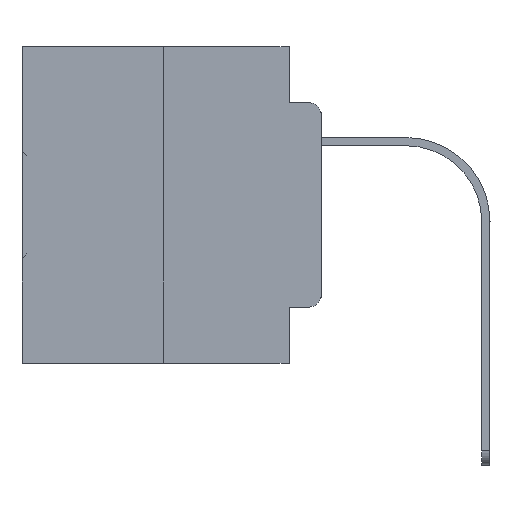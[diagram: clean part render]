
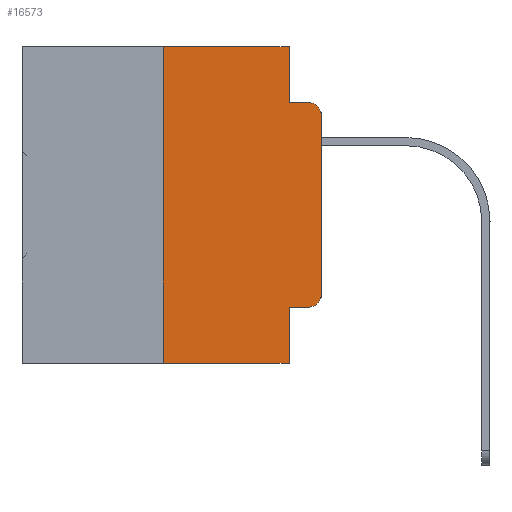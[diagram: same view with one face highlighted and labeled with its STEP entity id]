
A CAD part, left-side view. The second image highlights one B-rep face of the part: STEP entity #16573.
In plain terms, the highlighted planar face has unit normal (-1, 0, 0).
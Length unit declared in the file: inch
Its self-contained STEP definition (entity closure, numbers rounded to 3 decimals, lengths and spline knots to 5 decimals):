
#8 = ORIENTED_EDGE ( 'NONE', *, *, #15113, .F. ) ;
#86 = CIRCLE ( 'NONE', #32238, 0.02 ) ;
#237 = LINE ( 'NONE', #5363, #12974 ) ;
#696 = CARTESIAN_POINT ( 'NONE',  ( 0., 0.02, -0.1085 ) ) ;
#784 = VECTOR ( 'NONE', #29828, 39.37008 ) ;
#1221 = DIRECTION ( 'NONE',  ( -1., 0., 0. ) ) ;
#1241 = VERTEX_POINT ( 'NONE', #31182 ) ;
#1507 = VERTEX_POINT ( 'NONE', #30000 ) ;
#2081 = FACE_OUTER_BOUND ( 'NONE', #9160, .T. ) ;
#2321 = VECTOR ( 'NONE', #7804, 39.37008 ) ;
#2793 = EDGE_CURVE ( 'NONE', #11692, #13692, #12373, .T. ) ;
#2879 = ORIENTED_EDGE ( 'NONE', *, *, #31612, .T. ) ;
#3747 = DIRECTION ( 'NONE',  ( 0., 0., -1. ) ) ;
#4838 = AXIS2_PLACEMENT_3D ( 'NONE', #11300, #1221, #3747 ) ;
#5363 = CARTESIAN_POINT ( 'NONE',  ( 0., 0.051, -0.0885 ) ) ;
#6650 = CARTESIAN_POINT ( 'NONE',  ( 0., 0.25, 0. ) ) ;
#7146 = VECTOR ( 'NONE', #32523, 39.37008 ) ;
#7234 = DIRECTION ( 'NONE',  ( 0., 0., -1. ) ) ;
#7804 = DIRECTION ( 'NONE',  ( 0., -1., 0. ) ) ;
#9115 = CIRCLE ( 'NONE', #4838, 0.02 ) ;
#9160 = EDGE_LOOP ( 'NONE', ( #28665, #2879, #30508, #32165, #8, #24596, #19475, #17273, #24888, #32002 ) ) ;
#9454 = CARTESIAN_POINT ( 'NONE',  ( 0., 0.473, 0. ) ) ;
#10565 = CARTESIAN_POINT ( 'NONE',  ( 0., 0.02, -0.4115 ) ) ;
#10574 = DIRECTION ( 'NONE',  ( 0., -1., 0. ) ) ;
#10741 = VERTEX_POINT ( 'NONE', #19935 ) ;
#11232 = CARTESIAN_POINT ( 'NONE',  ( 0., 0.02, -0.0885 ) ) ;
#11300 = CARTESIAN_POINT ( 'NONE',  ( 0., 0.02, -0.3915 ) ) ;
#11692 = VERTEX_POINT ( 'NONE', #14006 ) ;
#12181 = CARTESIAN_POINT ( 'NONE',  ( 0., 0.051, -0.5 ) ) ;
#12209 = CARTESIAN_POINT ( 'NONE',  ( 0., 0.051, 0. ) ) ;
#12306 = DIRECTION ( 'NONE',  ( 1., 0., 0. ) ) ;
#12373 = LINE ( 'NONE', #12209, #7146 ) ;
#12952 = DIRECTION ( 'NONE',  ( -1., 0., 0. ) ) ;
#12974 = VECTOR ( 'NONE', #20783, 39.37008 ) ;
#13562 = CARTESIAN_POINT ( 'NONE',  ( 0., 0.473, 0. ) ) ;
#13692 = VERTEX_POINT ( 'NONE', #14424 ) ;
#14006 = CARTESIAN_POINT ( 'NONE',  ( 0., 0.051, 0. ) ) ;
#14424 = CARTESIAN_POINT ( 'NONE',  ( 0., 0.051, -0.0885 ) ) ;
#14685 = CARTESIAN_POINT ( 'NONE',  ( 0., 0.473, -0.5 ) ) ;
#14699 = LINE ( 'NONE', #6650, #784 ) ;
#14816 = CARTESIAN_POINT ( 'NONE',  ( 0., 0., 0. ) ) ;
#15113 = EDGE_CURVE ( 'NONE', #16890, #11692, #20601, .T. ) ;
#16573 = ADVANCED_FACE ( 'NONE', ( #2081 ), #27249, .F. ) ;
#16890 = VERTEX_POINT ( 'NONE', #25022 ) ;
#16979 = CARTESIAN_POINT ( 'NONE',  ( 0., 0.051, 0. ) ) ;
#17139 = LINE ( 'NONE', #16979, #17407 ) ;
#17257 = VERTEX_POINT ( 'NONE', #11232 ) ;
#17273 = ORIENTED_EDGE ( 'NONE', *, *, #19400, .F. ) ;
#17407 = VECTOR ( 'NONE', #7234, 39.37008 ) ;
#17802 = EDGE_CURVE ( 'NONE', #27132, #10741, #19677, .T. ) ;
#18368 = EDGE_CURVE ( 'NONE', #1241, #25806, #20458, .T. ) ;
#19094 = EDGE_CURVE ( 'NONE', #1507, #16890, #14699, .T. ) ;
#19400 = EDGE_CURVE ( 'NONE', #1241, #32311, #17139, .T. ) ;
#19475 = ORIENTED_EDGE ( 'NONE', *, *, #27829, .T. ) ;
#19677 = LINE ( 'NONE', #14816, #24809 ) ;
#19935 = CARTESIAN_POINT ( 'NONE',  ( 0., 0., -0.1085 ) ) ;
#20458 = LINE ( 'NONE', #20627, #29711 ) ;
#20601 = LINE ( 'NONE', #13562, #23354 ) ;
#20627 = CARTESIAN_POINT ( 'NONE',  ( 0., 0.051, -0.4115 ) ) ;
#20783 = DIRECTION ( 'NONE',  ( 0., -1., 0. ) ) ;
#23113 = DIRECTION ( 'NONE',  ( 0., -1., 0. ) ) ;
#23235 = AXIS2_PLACEMENT_3D ( 'NONE', #9454, #12306, #32770 ) ;
#23354 = VECTOR ( 'NONE', #23113, 39.37008 ) ;
#24596 = ORIENTED_EDGE ( 'NONE', *, *, #19094, .F. ) ;
#24809 = VECTOR ( 'NONE', #25065, 39.37008 ) ;
#24888 = ORIENTED_EDGE ( 'NONE', *, *, #18368, .T. ) ;
#25022 = CARTESIAN_POINT ( 'NONE',  ( 0., 0.25, 0. ) ) ;
#25065 = DIRECTION ( 'NONE',  ( 0., 0., 1. ) ) ;
#25806 = VERTEX_POINT ( 'NONE', #10565 ) ;
#26046 = CARTESIAN_POINT ( 'NONE',  ( 0., 0., -0.3915 ) ) ;
#27132 = VERTEX_POINT ( 'NONE', #26046 ) ;
#27249 = PLANE ( 'NONE',  #23235 ) ;
#27829 = EDGE_CURVE ( 'NONE', #1507, #32311, #30463, .T. ) ;
#28665 = ORIENTED_EDGE ( 'NONE', *, *, #17802, .T. ) ;
#29711 = VECTOR ( 'NONE', #10574, 39.37008 ) ;
#29828 = DIRECTION ( 'NONE',  ( 0., 0., 1. ) ) ;
#30000 = CARTESIAN_POINT ( 'NONE',  ( 0., 0.25, -0.5 ) ) ;
#30041 = EDGE_CURVE ( 'NONE', #25806, #27132, #9115, .T. ) ;
#30463 = LINE ( 'NONE', #14685, #2321 ) ;
#30508 = ORIENTED_EDGE ( 'NONE', *, *, #32036, .F. ) ;
#30752 = DIRECTION ( 'NONE',  ( 0., 0., -1. ) ) ;
#31182 = CARTESIAN_POINT ( 'NONE',  ( 0., 0.051, -0.4115 ) ) ;
#31612 = EDGE_CURVE ( 'NONE', #10741, #17257, #86, .T. ) ;
#32002 = ORIENTED_EDGE ( 'NONE', *, *, #30041, .T. ) ;
#32036 = EDGE_CURVE ( 'NONE', #13692, #17257, #237, .T. ) ;
#32165 = ORIENTED_EDGE ( 'NONE', *, *, #2793, .F. ) ;
#32238 = AXIS2_PLACEMENT_3D ( 'NONE', #696, #12952, #30752 ) ;
#32311 = VERTEX_POINT ( 'NONE', #12181 ) ;
#32523 = DIRECTION ( 'NONE',  ( 0., 0., -1. ) ) ;
#32770 = DIRECTION ( 'NONE',  ( 0., 0., -1. ) ) ;
